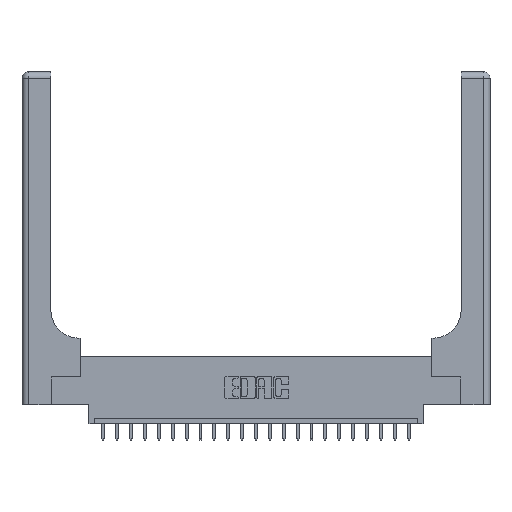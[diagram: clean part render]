
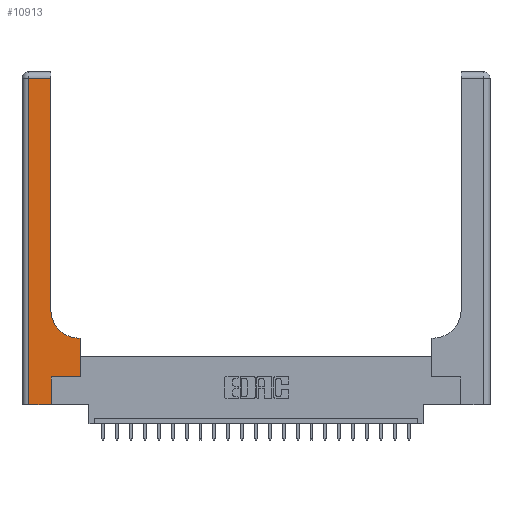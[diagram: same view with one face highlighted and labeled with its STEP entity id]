
A CAD part, top view. The second image highlights one B-rep face of the part: STEP entity #10913.
In plain terms, the highlighted planar face has unit normal (0, 0, 1).
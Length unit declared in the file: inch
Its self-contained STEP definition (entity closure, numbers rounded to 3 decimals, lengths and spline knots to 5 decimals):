
#1107 = VECTOR ( 'NONE', #7738, 39.37008 ) ;
#1444 = CARTESIAN_POINT ( 'NONE',  ( 0.26, 2.94, 0.37 ) ) ;
#1605 = CARTESIAN_POINT ( 'NONE',  ( 0.26, 3., 0.37 ) ) ;
#1994 = EDGE_CURVE ( 'NONE', #10797, #17673, #15299, .T. ) ;
#2332 = AXIS2_PLACEMENT_3D ( 'NONE', #21888, #2562, #13068 ) ;
#2562 = DIRECTION ( 'NONE',  ( 0., 0., -1. ) ) ;
#3199 = EDGE_CURVE ( 'NONE', #9018, #13051, #9997, .T. ) ;
#3963 = DIRECTION ( 'NONE',  ( 0., -1., 0. ) ) ;
#4043 = DIRECTION ( 'NONE',  ( 0., 0., -1. ) ) ;
#4751 = CARTESIAN_POINT ( 'NONE',  ( 0., 2.94, 0.37 ) ) ;
#5051 = DIRECTION ( 'NONE',  ( 1., 0., 0. ) ) ;
#5411 = VERTEX_POINT ( 'NONE', #14627 ) ;
#5501 = AXIS2_PLACEMENT_3D ( 'NONE', #5633, #4043, #18448 ) ;
#5633 = CARTESIAN_POINT ( 'NONE',  ( 0.51, 0.85, 0.37 ) ) ;
#5664 = ORIENTED_EDGE ( 'NONE', *, *, #8604, .T. ) ;
#5991 = CARTESIAN_POINT ( 'NONE',  ( 0.06, 0., 0.37 ) ) ;
#6200 = CARTESIAN_POINT ( 'NONE',  ( 0.265, 0.25, 0.37 ) ) ;
#6518 = LINE ( 'NONE', #17178, #14873 ) ;
#7053 = DIRECTION ( 'NONE',  ( 0., 1., 0. ) ) ;
#7479 = LINE ( 'NONE', #14236, #8680 ) ;
#7738 = DIRECTION ( 'NONE',  ( 0., 1., 0. ) ) ;
#7790 = ORIENTED_EDGE ( 'NONE', *, *, #10866, .T. ) ;
#7796 = EDGE_LOOP ( 'NONE', ( #5664, #22160, #18743, #8789, #15567, #7790, #13792, #22117, #10137 ) ) ;
#8143 = LINE ( 'NONE', #6200, #20952 ) ;
#8444 = VECTOR ( 'NONE', #17109, 39.37008 ) ;
#8446 = LINE ( 'NONE', #1605, #18513 ) ;
#8604 = EDGE_CURVE ( 'NONE', #13670, #18540, #8446, .T. ) ;
#8680 = VECTOR ( 'NONE', #3963, 39.37008 ) ;
#8789 = ORIENTED_EDGE ( 'NONE', *, *, #14832, .T. ) ;
#9018 = VERTEX_POINT ( 'NONE', #9675 ) ;
#9675 = CARTESIAN_POINT ( 'NONE',  ( 0.528, 0.6, 0.37 ) ) ;
#9997 = LINE ( 'NONE', #11719, #11134 ) ;
#10137 = ORIENTED_EDGE ( 'NONE', *, *, #20808, .T. ) ;
#10543 = CARTESIAN_POINT ( 'NONE',  ( 0.51, 0.6, 0.37 ) ) ;
#10797 = VERTEX_POINT ( 'NONE', #19604 ) ;
#10866 = EDGE_CURVE ( 'NONE', #17673, #5411, #8143, .T. ) ;
#10913 = ADVANCED_FACE ( 'NONE', ( #19947 ), #18127, .F. ) ;
#11115 = DIRECTION ( 'NONE',  ( 0., 1., 0. ) ) ;
#11134 = VECTOR ( 'NONE', #18727, 39.37008 ) ;
#11233 = CARTESIAN_POINT ( 'NONE',  ( 0.265, 0., 0.37 ) ) ;
#11719 = CARTESIAN_POINT ( 'NONE',  ( 0.26, 0.6, 0.37 ) ) ;
#12947 = DIRECTION ( 'NONE',  ( 1., 0., 0. ) ) ;
#13051 = VERTEX_POINT ( 'NONE', #10543 ) ;
#13068 = DIRECTION ( 'NONE',  ( -1., 0., 0. ) ) ;
#13670 = VERTEX_POINT ( 'NONE', #18961 ) ;
#13792 = ORIENTED_EDGE ( 'NONE', *, *, #19772, .T. ) ;
#14236 = CARTESIAN_POINT ( 'NONE',  ( 0.06, 3., 0.37 ) ) ;
#14627 = CARTESIAN_POINT ( 'NONE',  ( 0.528, 0.25, 0.37 ) ) ;
#14717 = CARTESIAN_POINT ( 'NONE',  ( 0.528, 0.25, 0.37 ) ) ;
#14832 = EDGE_CURVE ( 'NONE', #15636, #10797, #6518, .T. ) ;
#14873 = VECTOR ( 'NONE', #5051, 39.37008 ) ;
#15299 = LINE ( 'NONE', #11233, #16141 ) ;
#15567 = ORIENTED_EDGE ( 'NONE', *, *, #1994, .T. ) ;
#15636 = VERTEX_POINT ( 'NONE', #5991 ) ;
#16141 = VECTOR ( 'NONE', #11115, 39.37008 ) ;
#17109 = DIRECTION ( 'NONE',  ( -1., 0., 0. ) ) ;
#17178 = CARTESIAN_POINT ( 'NONE',  ( 0., 0., 0.37 ) ) ;
#17673 = VERTEX_POINT ( 'NONE', #21033 ) ;
#18127 = PLANE ( 'NONE',  #2332 ) ;
#18212 = EDGE_CURVE ( 'NONE', #21159, #15636, #7479, .T. ) ;
#18448 = DIRECTION ( 'NONE',  ( 1., 0., 0. ) ) ;
#18480 = LINE ( 'NONE', #4751, #8444 ) ;
#18513 = VECTOR ( 'NONE', #7053, 39.37008 ) ;
#18540 = VERTEX_POINT ( 'NONE', #1444 ) ;
#18727 = DIRECTION ( 'NONE',  ( -1., 0., 0. ) ) ;
#18743 = ORIENTED_EDGE ( 'NONE', *, *, #18212, .T. ) ;
#18961 = CARTESIAN_POINT ( 'NONE',  ( 0.26, 0.85, 0.37 ) ) ;
#19025 = CIRCLE ( 'NONE', #5501, 0.25 ) ;
#19604 = CARTESIAN_POINT ( 'NONE',  ( 0.265, 0., 0.37 ) ) ;
#19772 = EDGE_CURVE ( 'NONE', #5411, #9018, #21363, .T. ) ;
#19947 = FACE_OUTER_BOUND ( 'NONE', #7796, .T. ) ;
#20808 = EDGE_CURVE ( 'NONE', #13051, #13670, #19025, .T. ) ;
#20952 = VECTOR ( 'NONE', #12947, 39.37008 ) ;
#21033 = CARTESIAN_POINT ( 'NONE',  ( 0.265, 0.25, 0.37 ) ) ;
#21159 = VERTEX_POINT ( 'NONE', #21285 ) ;
#21285 = CARTESIAN_POINT ( 'NONE',  ( 0.06, 2.94, 0.37 ) ) ;
#21363 = LINE ( 'NONE', #14717, #1107 ) ;
#21756 = EDGE_CURVE ( 'NONE', #18540, #21159, #18480, .T. ) ;
#21888 = CARTESIAN_POINT ( 'NONE',  ( 0., 3., 0.37 ) ) ;
#22117 = ORIENTED_EDGE ( 'NONE', *, *, #3199, .T. ) ;
#22160 = ORIENTED_EDGE ( 'NONE', *, *, #21756, .T. ) ;
